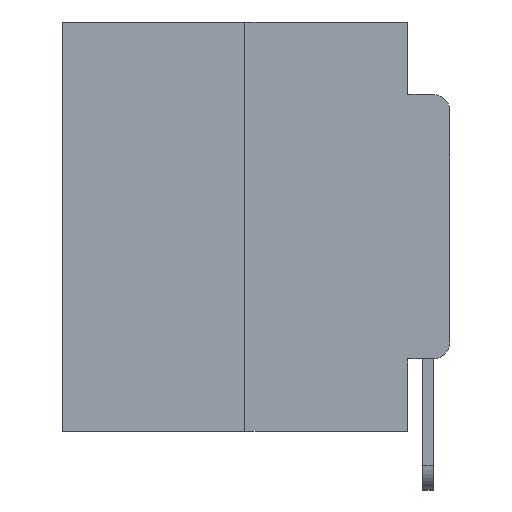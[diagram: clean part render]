
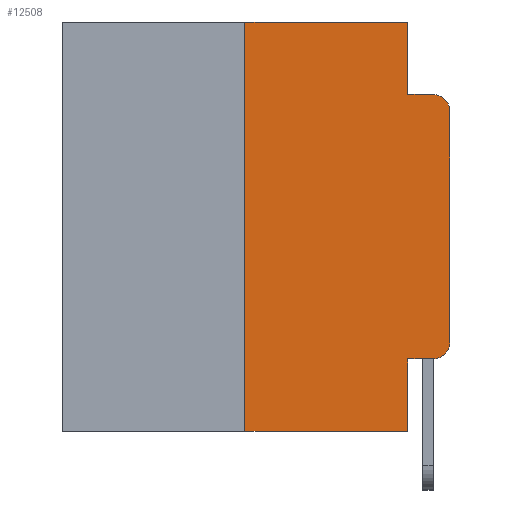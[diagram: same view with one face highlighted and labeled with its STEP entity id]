
A CAD part, left-side view. The second image highlights one B-rep face of the part: STEP entity #12508.
In plain terms, the highlighted planar face has unit normal (-1, 0, 0).
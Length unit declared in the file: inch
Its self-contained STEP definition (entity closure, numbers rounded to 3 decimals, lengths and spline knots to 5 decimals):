
#52 = DIRECTION ( 'NONE',  ( 0., 0., -1. ) ) ;
#747 = LINE ( 'NONE', #26280, #12201 ) ;
#1394 = VERTEX_POINT ( 'NONE', #26042 ) ;
#1544 = CIRCLE ( 'NONE', #18929, 0.02 ) ;
#1662 = CARTESIAN_POINT ( 'NONE',  ( 0., 0.02, -0.1085 ) ) ;
#2482 = CARTESIAN_POINT ( 'NONE',  ( 0., 0.473, 0. ) ) ;
#2569 = EDGE_CURVE ( 'NONE', #23280, #17200, #15677, .T. ) ;
#4044 = VECTOR ( 'NONE', #4630, 39.37008 ) ;
#4081 = DIRECTION ( 'NONE',  ( 0., 0., -1. ) ) ;
#4630 = DIRECTION ( 'NONE',  ( 0., -1., 0. ) ) ;
#4798 = LINE ( 'NONE', #22114, #20155 ) ;
#4899 = DIRECTION ( 'NONE',  ( 0., 0., -1. ) ) ;
#5720 = DIRECTION ( 'NONE',  ( 0., 0., -1. ) ) ;
#6079 = LINE ( 'NONE', #2482, #15991 ) ;
#6691 = ORIENTED_EDGE ( 'NONE', *, *, #19541, .F. ) ;
#7174 = CARTESIAN_POINT ( 'NONE',  ( 0., 0., 0. ) ) ;
#7777 = CARTESIAN_POINT ( 'NONE',  ( 0., 0.051, -0.0885 ) ) ;
#8477 = EDGE_CURVE ( 'NONE', #23280, #18383, #24101, .T. ) ;
#8932 = EDGE_CURVE ( 'NONE', #1394, #24877, #747, .T. ) ;
#9143 = AXIS2_PLACEMENT_3D ( 'NONE', #1662, #16933, #4081 ) ;
#9368 = CARTESIAN_POINT ( 'NONE',  ( 0., 0.25, 0. ) ) ;
#9604 = CARTESIAN_POINT ( 'NONE',  ( 0., 0.051, -0.4115 ) ) ;
#10303 = VECTOR ( 'NONE', #11925, 39.37008 ) ;
#10335 = EDGE_CURVE ( 'NONE', #24877, #19051, #14274, .T. ) ;
#10426 = VERTEX_POINT ( 'NONE', #9604 ) ;
#10635 = ORIENTED_EDGE ( 'NONE', *, *, #22251, .T. ) ;
#11109 = CARTESIAN_POINT ( 'NONE',  ( 0., 0., -0.3915 ) ) ;
#11573 = DIRECTION ( 'NONE',  ( 0., -1., 0. ) ) ;
#11925 = DIRECTION ( 'NONE',  ( 0., 0., 1. ) ) ;
#12201 = VECTOR ( 'NONE', #20574, 39.37008 ) ;
#12508 = ADVANCED_FACE ( 'NONE', ( #22722 ), #15581, .F. ) ;
#12550 = CARTESIAN_POINT ( 'NONE',  ( 0., 0.02, -0.0885 ) ) ;
#13090 = VECTOR ( 'NONE', #20857, 39.37008 ) ;
#13153 = ORIENTED_EDGE ( 'NONE', *, *, #8932, .F. ) ;
#13581 = DIRECTION ( 'NONE',  ( -1., 0., 0. ) ) ;
#14053 = CIRCLE ( 'NONE', #9143, 0.02 ) ;
#14274 = LINE ( 'NONE', #19348, #4044 ) ;
#14328 = ORIENTED_EDGE ( 'NONE', *, *, #2569, .F. ) ;
#15581 = PLANE ( 'NONE',  #20034 ) ;
#15677 = LINE ( 'NONE', #25599, #10303 ) ;
#15991 = VECTOR ( 'NONE', #11573, 39.37008 ) ;
#16230 = CARTESIAN_POINT ( 'NONE',  ( 0., 0.02, -0.4115 ) ) ;
#16239 = EDGE_CURVE ( 'NONE', #26177, #27042, #1544, .T. ) ;
#16455 = VERTEX_POINT ( 'NONE', #19997 ) ;
#16932 = ORIENTED_EDGE ( 'NONE', *, *, #20985, .T. ) ;
#16933 = DIRECTION ( 'NONE',  ( -1., 0., 0. ) ) ;
#17200 = VERTEX_POINT ( 'NONE', #9368 ) ;
#17615 = DIRECTION ( 'NONE',  ( 1., 0., 0. ) ) ;
#18383 = VERTEX_POINT ( 'NONE', #23675 ) ;
#18487 = CARTESIAN_POINT ( 'NONE',  ( 0., 0.25, -0.5 ) ) ;
#18678 = LINE ( 'NONE', #7174, #23145 ) ;
#18929 = AXIS2_PLACEMENT_3D ( 'NONE', #25274, #13581, #52 ) ;
#19051 = VERTEX_POINT ( 'NONE', #12550 ) ;
#19348 = CARTESIAN_POINT ( 'NONE',  ( 0., 0.051, -0.0885 ) ) ;
#19541 = EDGE_CURVE ( 'NONE', #17200, #1394, #6079, .T. ) ;
#19997 = CARTESIAN_POINT ( 'NONE',  ( 0., 0., -0.1085 ) ) ;
#20010 = ORIENTED_EDGE ( 'NONE', *, *, #10335, .F. ) ;
#20034 = AXIS2_PLACEMENT_3D ( 'NONE', #23301, #17615, #4899 ) ;
#20155 = VECTOR ( 'NONE', #5720, 39.37008 ) ;
#20574 = DIRECTION ( 'NONE',  ( 0., 0., -1. ) ) ;
#20857 = DIRECTION ( 'NONE',  ( 0., -1., 0. ) ) ;
#20985 = EDGE_CURVE ( 'NONE', #16455, #19051, #14053, .T. ) ;
#21354 = DIRECTION ( 'NONE',  ( 0., 0., 1. ) ) ;
#22114 = CARTESIAN_POINT ( 'NONE',  ( 0., 0.051, 0. ) ) ;
#22251 = EDGE_CURVE ( 'NONE', #27042, #16455, #18678, .T. ) ;
#22265 = CARTESIAN_POINT ( 'NONE',  ( 0., 0.051, -0.4115 ) ) ;
#22611 = ORIENTED_EDGE ( 'NONE', *, *, #22739, .T. ) ;
#22722 = FACE_OUTER_BOUND ( 'NONE', #26546, .T. ) ;
#22739 = EDGE_CURVE ( 'NONE', #10426, #26177, #24041, .T. ) ;
#23145 = VECTOR ( 'NONE', #21354, 39.37008 ) ;
#23280 = VERTEX_POINT ( 'NONE', #18487 ) ;
#23301 = CARTESIAN_POINT ( 'NONE',  ( 0., 0.473, 0. ) ) ;
#23675 = CARTESIAN_POINT ( 'NONE',  ( 0., 0.051, -0.5 ) ) ;
#24041 = LINE ( 'NONE', #22265, #26162 ) ;
#24101 = LINE ( 'NONE', #26636, #13090 ) ;
#24877 = VERTEX_POINT ( 'NONE', #7777 ) ;
#25274 = CARTESIAN_POINT ( 'NONE',  ( 0., 0.02, -0.3915 ) ) ;
#25330 = EDGE_CURVE ( 'NONE', #10426, #18383, #4798, .T. ) ;
#25599 = CARTESIAN_POINT ( 'NONE',  ( 0., 0.25, 0. ) ) ;
#26042 = CARTESIAN_POINT ( 'NONE',  ( 0., 0.051, 0. ) ) ;
#26142 = DIRECTION ( 'NONE',  ( 0., -1., 0. ) ) ;
#26162 = VECTOR ( 'NONE', #26142, 39.37008 ) ;
#26177 = VERTEX_POINT ( 'NONE', #16230 ) ;
#26199 = ORIENTED_EDGE ( 'NONE', *, *, #8477, .T. ) ;
#26280 = CARTESIAN_POINT ( 'NONE',  ( 0., 0.051, 0. ) ) ;
#26376 = ORIENTED_EDGE ( 'NONE', *, *, #16239, .T. ) ;
#26546 = EDGE_LOOP ( 'NONE', ( #10635, #16932, #20010, #13153, #6691, #14328, #26199, #27071, #22611, #26376 ) ) ;
#26636 = CARTESIAN_POINT ( 'NONE',  ( 0., 0.473, -0.5 ) ) ;
#27042 = VERTEX_POINT ( 'NONE', #11109 ) ;
#27071 = ORIENTED_EDGE ( 'NONE', *, *, #25330, .F. ) ;
